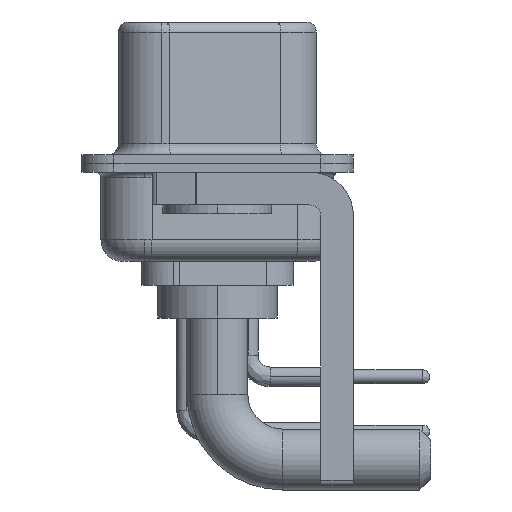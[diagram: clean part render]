
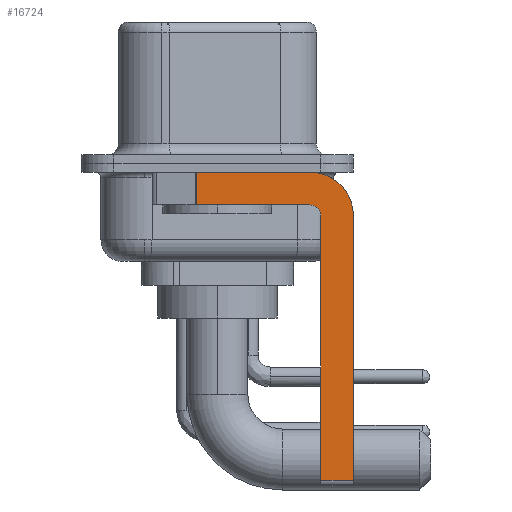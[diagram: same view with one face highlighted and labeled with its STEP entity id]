
A CAD part, left-side view. The second image highlights one B-rep face of the part: STEP entity #16724.
In plain terms, the highlighted planar face has unit normal (-1, 0, 0).
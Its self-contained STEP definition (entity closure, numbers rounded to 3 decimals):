
#171 = DIRECTION ( 'NONE',  ( 0., 0., -1. ) ) ;
#399 = DIRECTION ( 'NONE',  ( 0., 0., 1. ) ) ;
#788 = DIRECTION ( 'NONE',  ( -1., 0., 0. ) ) ;
#1026 = ORIENTED_EDGE ( 'NONE', *, *, #14332, .F. ) ;
#1049 = CARTESIAN_POINT ( 'NONE',  ( -2.9, -4.25, -2.4 ) ) ;
#1912 = CARTESIAN_POINT ( 'NONE',  ( -2.9, 0.978, -0.4 ) ) ;
#2631 = ORIENTED_EDGE ( 'NONE', *, *, #21489, .F. ) ;
#2633 = CARTESIAN_POINT ( 'NONE',  ( -2.9, -4.75, -14.8 ) ) ;
#2654 = CARTESIAN_POINT ( 'NONE',  ( -2.9, -4.25, -2.4 ) ) ;
#3098 = DIRECTION ( 'NONE',  ( 0., -1., 0. ) ) ;
#3728 = EDGE_CURVE ( 'NONE', #23326, #18944, #6600, .T. ) ;
#4163 = LINE ( 'NONE', #2633, #4995 ) ;
#4228 = ORIENTED_EDGE ( 'NONE', *, *, #20237, .T. ) ;
#4520 = AXIS2_PLACEMENT_3D ( 'NONE', #2654, #788, #399 ) ;
#4995 = VECTOR ( 'NONE', #25196, 1000. ) ;
#5942 = DIRECTION ( 'NONE',  ( 0., 0., -1. ) ) ;
#6316 = PLANE ( 'NONE',  #19058 ) ;
#6370 = EDGE_CURVE ( 'NONE', #20548, #22402, #4163, .T. ) ;
#6600 = CIRCLE ( 'NONE', #21519, 2. ) ;
#8058 = DIRECTION ( 'NONE',  ( 1., 0., 0. ) ) ;
#8064 = CARTESIAN_POINT ( 'NONE',  ( -2.9, -4.25, -0.4 ) ) ;
#8095 = CARTESIAN_POINT ( 'NONE',  ( -2.9, 0.978, -1.9 ) ) ;
#8229 = CARTESIAN_POINT ( 'NONE',  ( -2.9, -6.25, -2.4 ) ) ;
#9217 = DIRECTION ( 'NONE',  ( 1., 0., 0. ) ) ;
#9709 = VERTEX_POINT ( 'NONE', #25863 ) ;
#10308 = VECTOR ( 'NONE', #5942, 1000. ) ;
#11355 = VERTEX_POINT ( 'NONE', #1912 ) ;
#11805 = CARTESIAN_POINT ( 'NONE',  ( -2.9, -4.75, -14.55 ) ) ;
#12206 = CARTESIAN_POINT ( 'NONE',  ( -2.9, -4.25, -2.4 ) ) ;
#12233 = CARTESIAN_POINT ( 'NONE',  ( -2.9, 0.978, -1.9 ) ) ;
#12651 = DIRECTION ( 'NONE',  ( 0., 1., 0. ) ) ;
#13032 = VECTOR ( 'NONE', #3098, 1000. ) ;
#13933 = CARTESIAN_POINT ( 'NONE',  ( -2.9, 3., -0.4 ) ) ;
#14196 = CARTESIAN_POINT ( 'NONE',  ( -2.9, -6.25, -14.55 ) ) ;
#14332 = EDGE_CURVE ( 'NONE', #22402, #9709, #23670, .T. ) ;
#14643 = DIRECTION ( 'NONE',  ( 0., 0., -1. ) ) ;
#14649 = CARTESIAN_POINT ( 'NONE',  ( -2.9, -4.75, -2.4 ) ) ;
#15350 = ORIENTED_EDGE ( 'NONE', *, *, #16760, .F. ) ;
#15367 = DIRECTION ( 'NONE',  ( 0., 0., -1. ) ) ;
#15652 = VECTOR ( 'NONE', #12651, 1000. ) ;
#16663 = CARTESIAN_POINT ( 'NONE',  ( -2.9, -4.25, -1.9 ) ) ;
#16724 = ADVANCED_FACE ( 'NONE', ( #24469 ), #6316, .F. ) ;
#16735 = VERTEX_POINT ( 'NONE', #14196 ) ;
#16760 = EDGE_CURVE ( 'NONE', #11355, #23326, #22469, .T. ) ;
#17807 = CARTESIAN_POINT ( 'NONE',  ( -2.9, -4.25, -14.55 ) ) ;
#18077 = ORIENTED_EDGE ( 'NONE', *, *, #6370, .F. ) ;
#18384 = LINE ( 'NONE', #8229, #22732 ) ;
#18944 = VERTEX_POINT ( 'NONE', #20277 ) ;
#19058 = AXIS2_PLACEMENT_3D ( 'NONE', #12206, #8058, #171 ) ;
#19460 = VECTOR ( 'NONE', #22331, 1000. ) ;
#20237 = EDGE_CURVE ( 'NONE', #11355, #22247, #24769, .T. ) ;
#20277 = CARTESIAN_POINT ( 'NONE',  ( -2.9, -6.25, -2.4 ) ) ;
#20548 = VERTEX_POINT ( 'NONE', #11805 ) ;
#21489 = EDGE_CURVE ( 'NONE', #18944, #16735, #18384, .T. ) ;
#21519 = AXIS2_PLACEMENT_3D ( 'NONE', #1049, #9217, #15367 ) ;
#22247 = VERTEX_POINT ( 'NONE', #8095 ) ;
#22331 = DIRECTION ( 'NONE',  ( 0., -1., 0. ) ) ;
#22402 = VERTEX_POINT ( 'NONE', #14649 ) ;
#22469 = LINE ( 'NONE', #13933, #19460 ) ;
#22637 = LINE ( 'NONE', #16663, #15652 ) ;
#22732 = VECTOR ( 'NONE', #14643, 1000. ) ;
#23326 = VERTEX_POINT ( 'NONE', #8064 ) ;
#23513 = ORIENTED_EDGE ( 'NONE', *, *, #3728, .F. ) ;
#23653 = LINE ( 'NONE', #17807, #13032 ) ;
#23670 = CIRCLE ( 'NONE', #4520, 0.5 ) ;
#23702 = EDGE_CURVE ( 'NONE', #20548, #16735, #23653, .T. ) ;
#23849 = ORIENTED_EDGE ( 'NONE', *, *, #23702, .T. ) ;
#24469 = FACE_OUTER_BOUND ( 'NONE', #25438, .T. ) ;
#24769 = LINE ( 'NONE', #12233, #10308 ) ;
#24799 = ORIENTED_EDGE ( 'NONE', *, *, #26201, .F. ) ;
#25196 = DIRECTION ( 'NONE',  ( 0., 0., 1. ) ) ;
#25438 = EDGE_LOOP ( 'NONE', ( #15350, #4228, #24799, #1026, #18077, #23849, #2631, #23513 ) ) ;
#25863 = CARTESIAN_POINT ( 'NONE',  ( -2.9, -4.25, -1.9 ) ) ;
#26201 = EDGE_CURVE ( 'NONE', #9709, #22247, #22637, .T. ) ;
